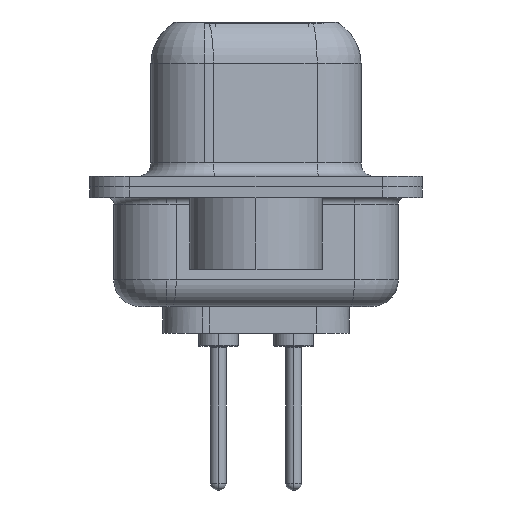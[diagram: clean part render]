
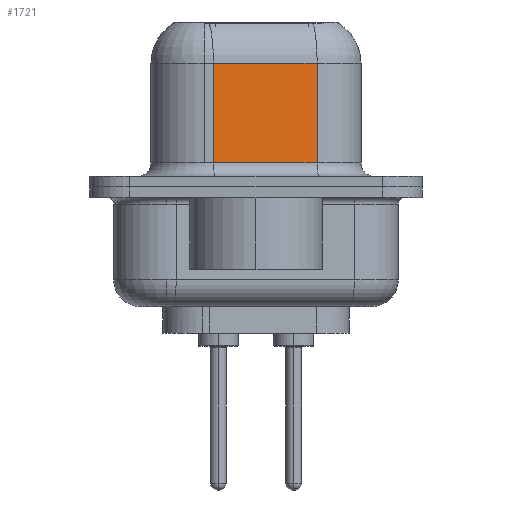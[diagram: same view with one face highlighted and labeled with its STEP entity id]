
A CAD part, left-side view. The second image highlights one B-rep face of the part: STEP entity #1721.
In plain terms, the highlighted planar face has unit normal (-0.985, -0.174, 0).
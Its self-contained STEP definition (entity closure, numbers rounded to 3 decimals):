
#644 = CARTESIAN_POINT ( 'NONE',  ( 5.068, -2.297, 6.4 ) ) ;
#737 = ORIENTED_EDGE ( 'NONE', *, *, #17834, .T. ) ;
#838 = EDGE_CURVE ( 'NONE', #14877, #9924, #8742, .T. ) ;
#906 = VERTEX_POINT ( 'NONE', #3946 ) ;
#1721 = ADVANCED_FACE ( 'NONE', ( #5789 ), #14584, .F. ) ;
#1846 = AXIS2_PLACEMENT_3D ( 'NONE', #644, #8850, #2175 ) ;
#2175 = DIRECTION ( 'NONE',  ( -0.174, 0.985, 0. ) ) ;
#3945 = CARTESIAN_POINT ( 'NONE',  ( 5.068, -2.297, 0.9 ) ) ;
#3946 = CARTESIAN_POINT ( 'NONE',  ( 4.38, 1.603, 0.9 ) ) ;
#4454 = CARTESIAN_POINT ( 'NONE',  ( 4.38, 1.603, 4.65 ) ) ;
#5508 = VECTOR ( 'NONE', #15724, 1000. ) ;
#5789 = FACE_OUTER_BOUND ( 'NONE', #9465, .T. ) ;
#6225 = CARTESIAN_POINT ( 'NONE',  ( 5.068, -2.297, 0.9 ) ) ;
#7060 = ORIENTED_EDGE ( 'NONE', *, *, #9415, .F. ) ;
#7534 = LINE ( 'NONE', #12899, #15926 ) ;
#8742 = LINE ( 'NONE', #14475, #5508 ) ;
#8850 = DIRECTION ( 'NONE',  ( 0.985, 0.174, 0. ) ) ;
#9415 = EDGE_CURVE ( 'NONE', #14877, #10660, #7534, .T. ) ;
#9465 = EDGE_LOOP ( 'NONE', ( #7060, #11548, #737, #16018 ) ) ;
#9924 = VERTEX_POINT ( 'NONE', #4454 ) ;
#10660 = VERTEX_POINT ( 'NONE', #3945 ) ;
#10905 = DIRECTION ( 'NONE',  ( 0., 0., -1. ) ) ;
#11548 = ORIENTED_EDGE ( 'NONE', *, *, #838, .T. ) ;
#12271 = LINE ( 'NONE', #17781, #13480 ) ;
#12808 = EDGE_CURVE ( 'NONE', #906, #10660, #16023, .T. ) ;
#12899 = CARTESIAN_POINT ( 'NONE',  ( 5.068, -2.297, 6.4 ) ) ;
#12926 = CARTESIAN_POINT ( 'NONE',  ( 5.068, -2.297, 4.65 ) ) ;
#13480 = VECTOR ( 'NONE', #10905, 1000. ) ;
#14182 = DIRECTION ( 'NONE',  ( 0., 0., -1. ) ) ;
#14475 = CARTESIAN_POINT ( 'NONE',  ( 5.068, -2.297, 4.65 ) ) ;
#14584 = PLANE ( 'NONE',  #1846 ) ;
#14877 = VERTEX_POINT ( 'NONE', #12926 ) ;
#14947 = VECTOR ( 'NONE', #17289, 1000. ) ;
#15724 = DIRECTION ( 'NONE',  ( -0.174, 0.985, 0. ) ) ;
#15926 = VECTOR ( 'NONE', #14182, 1000. ) ;
#16018 = ORIENTED_EDGE ( 'NONE', *, *, #12808, .T. ) ;
#16023 = LINE ( 'NONE', #6225, #14947 ) ;
#17289 = DIRECTION ( 'NONE',  ( 0.174, -0.985, 0. ) ) ;
#17781 = CARTESIAN_POINT ( 'NONE',  ( 4.38, 1.603, 6.4 ) ) ;
#17834 = EDGE_CURVE ( 'NONE', #9924, #906, #12271, .T. ) ;
